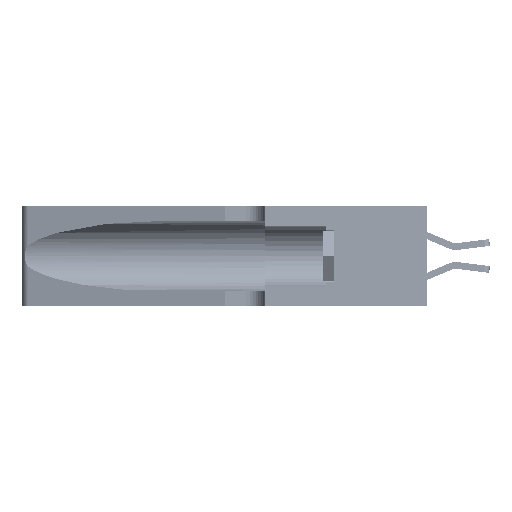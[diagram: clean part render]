
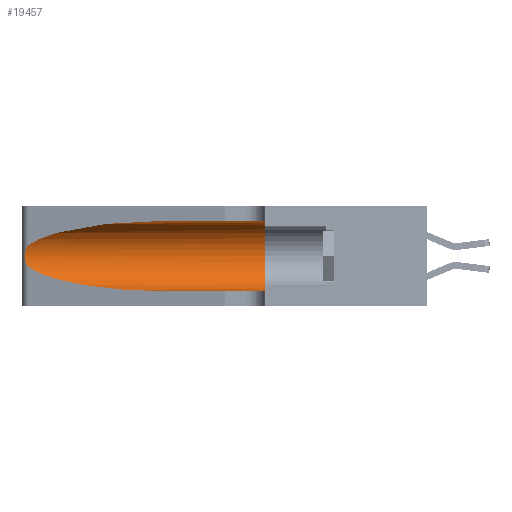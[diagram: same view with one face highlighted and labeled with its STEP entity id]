
A CAD part, left-side view. The second image highlights one B-rep face of the part: STEP entity #19457.
In plain terms, the highlighted cylindrical face has radius 3.308 mm (diameter 6.617 mm), a partial arc.
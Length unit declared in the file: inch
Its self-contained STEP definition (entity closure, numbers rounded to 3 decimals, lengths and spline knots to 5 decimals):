
#670 = VERTEX_POINT ( 'NONE', #20709 ) ;
#1102 = CARTESIAN_POINT ( 'NONE',  ( 0.25487, 1.22718, 0.14631 ) ) ;
#1657 = EDGE_CURVE ( 'NONE', #2631, #27617, #35982, .T. ) ;
#1944 = FACE_OUTER_BOUND ( 'NONE', #24328, .T. ) ;
#2631 = VERTEX_POINT ( 'NONE', #23858 ) ;
#2660 = DIRECTION ( 'NONE',  ( 0., 1., 0. ) ) ;
#3640 = CARTESIAN_POINT ( 'NONE',  ( 0.26075, 1.23896, 0.178 ) ) ;
#5485 = CARTESIAN_POINT ( 'NONE',  ( 0.25487, 1.22718, 0.14631 ) ) ;
#7348 = CARTESIAN_POINT ( 'NONE',  ( 0.25555, 1.22994, 0.2215 ) ) ;
#7367 = EDGE_CURVE ( 'NONE', #19765, #27617, #39335, .T. ) ;
#7507 = CARTESIAN_POINT ( 'NONE',  ( 0.25856, 1.23593, 0.16098 ) ) ;
#10248 = B_SPLINE_CURVE_WITH_KNOTS ( 'NONE', 3,
 ( #33849, #7348, #18817, #45184, #22631, #48940, #26428, #3640, #30247, #7507, #34010, #11368, #37798, #15201 ),
 .UNSPECIFIED., .F., .F.,
 ( 4, 2, 2, 2, 2, 2, 4 ),
 ( 0., 0.00027, 0.00053, 0.00107, 0.0016, 0.00187, 0.00214 ),
 .UNSPECIFIED. ) ;
#10286 = EDGE_CURVE ( 'NONE', #44421, #2631, #19061, .T. ) ;
#11368 = CARTESIAN_POINT ( 'NONE',  ( 0.25639, 1.23186, 0.15144 ) ) ;
#12028 = ORIENTED_EDGE ( 'NONE', *, *, #14759, .T. ) ;
#12889 = CARTESIAN_POINT ( 'NONE',  ( 0.18966, 0.96281, 0.31525 ) ) ;
#13240 = CARTESIAN_POINT ( 'NONE',  ( 0.1305, 0.72297, 0.05475 ) ) ;
#14759 = EDGE_CURVE ( 'NONE', #24825, #44421, #10248, .T. ) ;
#14775 = LINE ( 'NONE', #41484, #44845 ) ;
#15201 = CARTESIAN_POINT ( 'NONE',  ( 0.25487, 1.22718, 0.14631 ) ) ;
#15758 = DIRECTION ( 'NONE',  ( 0., -1., 0. ) ) ;
#15882 = VECTOR ( 'NONE', #40573, 39.37008 ) ;
#17979 = CARTESIAN_POINT ( 'NONE',  ( 0.1305, 1.61858, 0.05475 ) ) ;
#18817 = CARTESIAN_POINT ( 'NONE',  ( 0.25639, 1.23184, 0.21858 ) ) ;
#19061 =( BOUNDED_CURVE ( )  B_SPLINE_CURVE ( 3, ( #5485, #28276, #35849, #13240 ),
 .UNSPECIFIED., .F., .T. ) 
 B_SPLINE_CURVE_WITH_KNOTS ( ( 4, 4 ),
 ( 3.44316, 4.71239 ),
 .UNSPECIFIED. ) 
 CURVE ( )  GEOMETRIC_REPRESENTATION_ITEM ( )  RATIONAL_B_SPLINE_CURVE ( ( 1., 0.87, 0.87, 1. ) ) 
 REPRESENTATION_ITEM ( '' )  );
#19386 = ORIENTED_EDGE ( 'NONE', *, *, #40542, .F. ) ;
#19457 = ADVANCED_FACE ( 'NONE', ( #1944 ), #19866, .F. ) ;
#19765 = VERTEX_POINT ( 'NONE', #39984 ) ;
#19866 = CYLINDRICAL_SURFACE ( 'NONE', #43129, 0.13025 ) ;
#20709 = CARTESIAN_POINT ( 'NONE',  ( 0.1305, 0.72297, 0.31525 ) ) ;
#22631 = CARTESIAN_POINT ( 'NONE',  ( 0.25854, 1.2359, 0.20912 ) ) ;
#23192 = DIRECTION ( 'NONE',  ( 0., 0., -1. ) ) ;
#23352 = ORIENTED_EDGE ( 'NONE', *, *, #1657, .T. ) ;
#23858 = CARTESIAN_POINT ( 'NONE',  ( 0.1305, 0.72297, 0.05475 ) ) ;
#24281 = CARTESIAN_POINT ( 'NONE',  ( 0.25487, 1.22718, 0.22369 ) ) ;
#24328 = EDGE_LOOP ( 'NONE', ( #46797, #12028, #29222, #23352, #30088, #19386 ) ) ;
#24825 = VERTEX_POINT ( 'NONE', #41367 ) ;
#25479 = CARTESIAN_POINT ( 'NONE',  ( 0.1305, 0.35, 0.185 ) ) ;
#26428 = CARTESIAN_POINT ( 'NONE',  ( 0.26075, 1.23896, 0.19203 ) ) ;
#27617 = VERTEX_POINT ( 'NONE', #40622 ) ;
#28013 = EDGE_CURVE ( 'NONE', #670, #24825, #46837, .T. ) ;
#28276 = CARTESIAN_POINT ( 'NONE',  ( 0.2373, 1.15595, 0.08982 ) ) ;
#29222 = ORIENTED_EDGE ( 'NONE', *, *, #10286, .T. ) ;
#29287 = DIRECTION ( 'NONE',  ( 0., 0., 1. ) ) ;
#30088 = ORIENTED_EDGE ( 'NONE', *, *, #7367, .F. ) ;
#30247 = CARTESIAN_POINT ( 'NONE',  ( 0.26017, 1.23833, 0.17102 ) ) ;
#33849 = CARTESIAN_POINT ( 'NONE',  ( 0.25487, 1.22718, 0.22369 ) ) ;
#34010 = CARTESIAN_POINT ( 'NONE',  ( 0.25789, 1.23486, 0.15765 ) ) ;
#34572 = CARTESIAN_POINT ( 'NONE',  ( 0.1305, 1.61858, 0.185 ) ) ;
#34927 = AXIS2_PLACEMENT_3D ( 'NONE', #25479, #2660, #29287 ) ;
#35849 = CARTESIAN_POINT ( 'NONE',  ( 0.18966, 0.96281, 0.05475 ) ) ;
#35982 = LINE ( 'NONE', #17979, #15882 ) ;
#37798 = CARTESIAN_POINT ( 'NONE',  ( 0.25555, 1.22993, 0.14849 ) ) ;
#39262 = CARTESIAN_POINT ( 'NONE',  ( 0.1305, 0.72297, 0.31525 ) ) ;
#39335 = CIRCLE ( 'NONE', #34927, 0.13025 ) ;
#39984 = CARTESIAN_POINT ( 'NONE',  ( 0.1305, 0.35, 0.31525 ) ) ;
#40542 = EDGE_CURVE ( 'NONE', #670, #19765, #14775, .T. ) ;
#40573 = DIRECTION ( 'NONE',  ( 0., -1., 0. ) ) ;
#40622 = CARTESIAN_POINT ( 'NONE',  ( 0.1305, 0.35, 0.05475 ) ) ;
#41367 = CARTESIAN_POINT ( 'NONE',  ( 0.25487, 1.22718, 0.22369 ) ) ;
#41484 = CARTESIAN_POINT ( 'NONE',  ( 0.1305, 1.61858, 0.31525 ) ) ;
#43129 = AXIS2_PLACEMENT_3D ( 'NONE', #34572, #15758, #23192 ) ;
#44421 = VERTEX_POINT ( 'NONE', #1102 ) ;
#44845 = VECTOR ( 'NONE', #45261, 39.37008 ) ;
#45184 = CARTESIAN_POINT ( 'NONE',  ( 0.25787, 1.23484, 0.2124 ) ) ;
#45261 = DIRECTION ( 'NONE',  ( 0., -1., 0. ) ) ;
#46797 = ORIENTED_EDGE ( 'NONE', *, *, #28013, .T. ) ;
#46812 = CARTESIAN_POINT ( 'NONE',  ( 0.2373, 1.15595, 0.28018 ) ) ;
#46837 =( BOUNDED_CURVE ( )  B_SPLINE_CURVE ( 3, ( #39262, #12889, #46812, #24281 ),
 .UNSPECIFIED., .F., .F. ) 
 B_SPLINE_CURVE_WITH_KNOTS ( ( 4, 4 ),
 ( 1.5708, 2.84003 ),
 .UNSPECIFIED. ) 
 CURVE ( )  GEOMETRIC_REPRESENTATION_ITEM ( )  RATIONAL_B_SPLINE_CURVE ( ( 1., 0.87, 0.87, 1. ) ) 
 REPRESENTATION_ITEM ( '' )  );
#48940 = CARTESIAN_POINT ( 'NONE',  ( 0.26018, 1.23835, 0.19895 ) ) ;
